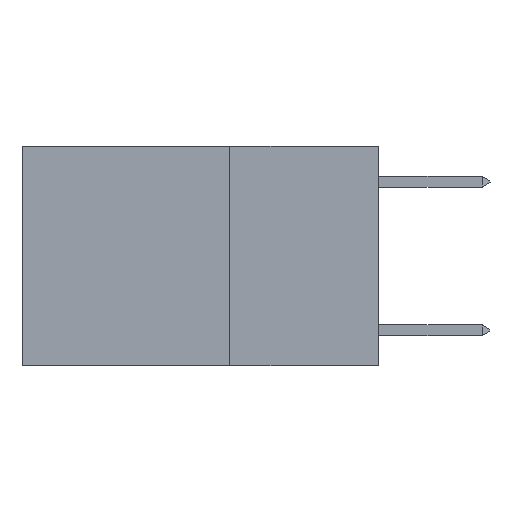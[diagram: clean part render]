
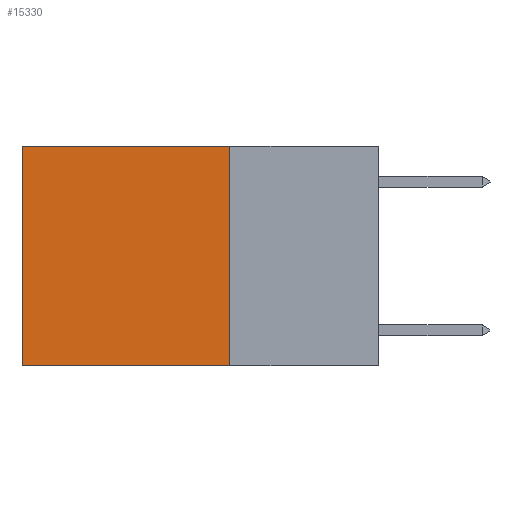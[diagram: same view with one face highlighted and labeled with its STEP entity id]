
A CAD part, left-side view. The second image highlights one B-rep face of the part: STEP entity #15330.
In plain terms, the highlighted planar face has unit normal (-1, 0, 0).
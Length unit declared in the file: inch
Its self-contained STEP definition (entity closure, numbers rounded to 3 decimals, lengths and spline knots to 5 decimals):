
#338 = DIRECTION ( 'NONE',  ( 1., 0., 0. ) ) ;
#547 = VERTEX_POINT ( 'NONE', #3393 ) ;
#1988 = EDGE_CURVE ( 'NONE', #3859, #15181, #2372, .T. ) ;
#2275 = DIRECTION ( 'NONE',  ( 0., 0., -1. ) ) ;
#2372 = LINE ( 'NONE', #12319, #14739 ) ;
#2630 = CARTESIAN_POINT ( 'NONE',  ( 0.2625, 0.25, 0. ) ) ;
#2798 = LINE ( 'NONE', #16690, #6252 ) ;
#3393 = CARTESIAN_POINT ( 'NONE',  ( 0.2625, 0.6, -0.37 ) ) ;
#3859 = VERTEX_POINT ( 'NONE', #2630 ) ;
#4543 = ORIENTED_EDGE ( 'NONE', *, *, #1988, .F. ) ;
#5390 = DIRECTION ( 'NONE',  ( 0., 1., 0. ) ) ;
#5647 = DIRECTION ( 'NONE',  ( 0., 1., 0. ) ) ;
#5834 = VERTEX_POINT ( 'NONE', #14266 ) ;
#6010 = ORIENTED_EDGE ( 'NONE', *, *, #10239, .T. ) ;
#6252 = VECTOR ( 'NONE', #5390, 39.37008 ) ;
#6594 = LINE ( 'NONE', #9186, #9736 ) ;
#6619 = CARTESIAN_POINT ( 'NONE',  ( 0.2625, 0.25, -0.37 ) ) ;
#6851 = EDGE_CURVE ( 'NONE', #5834, #547, #6594, .T. ) ;
#6970 = EDGE_CURVE ( 'NONE', #15181, #547, #2798, .T. ) ;
#9080 = VECTOR ( 'NONE', #5647, 39.37008 ) ;
#9186 = CARTESIAN_POINT ( 'NONE',  ( 0.2625, 0.6, 0. ) ) ;
#9736 = VECTOR ( 'NONE', #11847, 39.37008 ) ;
#10031 = DIRECTION ( 'NONE',  ( 0., 0., -1. ) ) ;
#10239 = EDGE_CURVE ( 'NONE', #3859, #5834, #12826, .T. ) ;
#10746 = ORIENTED_EDGE ( 'NONE', *, *, #6851, .T. ) ;
#11773 = AXIS2_PLACEMENT_3D ( 'NONE', #16889, #338, #10031 ) ;
#11847 = DIRECTION ( 'NONE',  ( 0., 0., -1. ) ) ;
#12319 = CARTESIAN_POINT ( 'NONE',  ( 0.2625, 0.25, 0. ) ) ;
#12826 = LINE ( 'NONE', #14018, #9080 ) ;
#12867 = FACE_OUTER_BOUND ( 'NONE', #15266, .T. ) ;
#14018 = CARTESIAN_POINT ( 'NONE',  ( 0.2625, 0.25, 0. ) ) ;
#14266 = CARTESIAN_POINT ( 'NONE',  ( 0.2625, 0.6, 0. ) ) ;
#14739 = VECTOR ( 'NONE', #2275, 39.37008 ) ;
#15181 = VERTEX_POINT ( 'NONE', #6619 ) ;
#15223 = ORIENTED_EDGE ( 'NONE', *, *, #6970, .F. ) ;
#15266 = EDGE_LOOP ( 'NONE', ( #10746, #15223, #4543, #6010 ) ) ;
#15330 = ADVANCED_FACE ( 'NONE', ( #12867 ), #17068, .F. ) ;
#16690 = CARTESIAN_POINT ( 'NONE',  ( 0.2625, 0.25, -0.37 ) ) ;
#16889 = CARTESIAN_POINT ( 'NONE',  ( 0.2625, 0.25, 0. ) ) ;
#17068 = PLANE ( 'NONE',  #11773 ) ;
